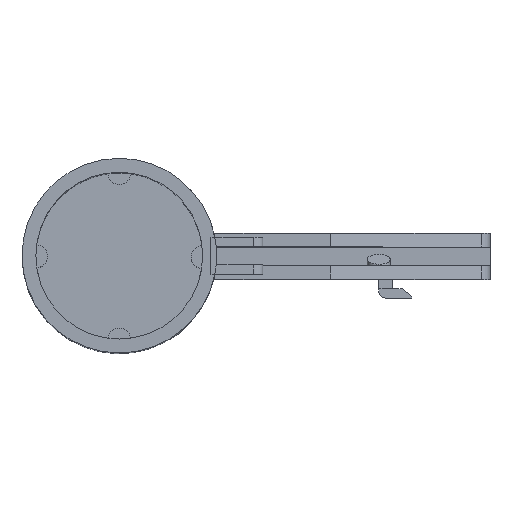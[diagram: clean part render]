
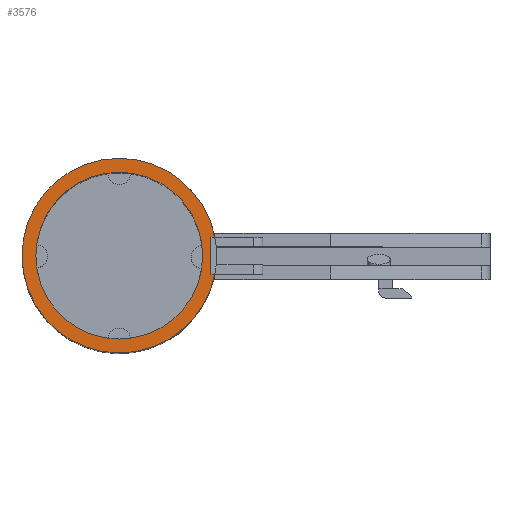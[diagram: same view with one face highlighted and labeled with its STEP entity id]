
A CAD part, top view. The second image highlights one B-rep face of the part: STEP entity #3576.
In plain terms, the highlighted planar face has unit normal (0, 0, 1).
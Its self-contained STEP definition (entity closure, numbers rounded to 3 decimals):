
#984 = CYLINDRICAL_SURFACE('',#985,21.);
#985 = AXIS2_PLACEMENT_3D('',#986,#987,#988);
#986 = CARTESIAN_POINT('',(0.,0.,0.));
#987 = DIRECTION('',(0.,0.,-1.));
#988 = DIRECTION('',(1.,0.,0.));
#2162 = VERTEX_POINT('',#2163);
#2163 = CARTESIAN_POINT('',(20.616,4.,100.));
#2187 = EDGE_CURVE('',#2162,#2188,#2190,.T.);
#2188 = VERTEX_POINT('',#2189);
#2189 = CARTESIAN_POINT('',(20.616,-4.,100.));
#2190 = SURFACE_CURVE('',#2191,(#2196,#2203),.PCURVE_S1.);
#2191 = CIRCLE('',#2192,21.);
#2192 = AXIS2_PLACEMENT_3D('',#2193,#2194,#2195);
#2193 = CARTESIAN_POINT('',(0.,0.,100.));
#2194 = DIRECTION('',(0.,0.,1.));
#2195 = DIRECTION('',(1.,0.,0.));
#2196 = PCURVE('',#984,#2197);
#2197 = DEFINITIONAL_REPRESENTATION('',(#2198),#2202);
#2198 = LINE('',#2199,#2200);
#2199 = CARTESIAN_POINT('',(0.,-100.));
#2200 = VECTOR('',#2201,1.);
#2201 = DIRECTION('',(-1.,0.));
#2202 = ( GEOMETRIC_REPRESENTATION_CONTEXT(2) 
PARAMETRIC_REPRESENTATION_CONTEXT() REPRESENTATION_CONTEXT('2D SPACE',''
  ) );
#2203 = PCURVE('',#2204,#2209);
#2204 = PLANE('',#2205);
#2205 = AXIS2_PLACEMENT_3D('',#2206,#2207,#2208);
#2206 = CARTESIAN_POINT('',(21.,0.,100.));
#2207 = DIRECTION('',(0.,0.,-1.));
#2208 = DIRECTION('',(-1.,0.,0.));
#2209 = DEFINITIONAL_REPRESENTATION('',(#2210),#2218);
#2210 = ( BOUNDED_CURVE() B_SPLINE_CURVE(2,(#2211,#2212,#2213,#2214,
#2215,#2216,#2217),.UNSPECIFIED.,.F.,.F.) B_SPLINE_CURVE_WITH_KNOTS((1,2
    ,2,2,2,1),(-2.094,0.,2.094,4.189,
6.283,8.378),.UNSPECIFIED.) CURVE() 
GEOMETRIC_REPRESENTATION_ITEM() RATIONAL_B_SPLINE_CURVE((1.,0.5,1.,0.5,
1.,0.5,1.)) REPRESENTATION_ITEM('') );
#2211 = CARTESIAN_POINT('',(0.,0.));
#2212 = CARTESIAN_POINT('',(0.,36.373));
#2213 = CARTESIAN_POINT('',(31.5,18.187));
#2214 = CARTESIAN_POINT('',(63.,0.));
#2215 = CARTESIAN_POINT('',(31.5,-18.187));
#2216 = CARTESIAN_POINT('',(0.,-36.373));
#2217 = CARTESIAN_POINT('',(0.,0.));
#2218 = ( GEOMETRIC_REPRESENTATION_CONTEXT(2) 
PARAMETRIC_REPRESENTATION_CONTEXT() REPRESENTATION_CONTEXT('2D SPACE',''
  ) );
#3576 = ADVANCED_FACE('',(#3577,#3652),#2204,.F.);
#3577 = FACE_BOUND('',#3578,.F.);
#3578 = EDGE_LOOP('',(#3579,#3580,#3608,#3631));
#3579 = ORIENTED_EDGE('',*,*,#2187,.F.);
#3580 = ORIENTED_EDGE('',*,*,#3581,.F.);
#3581 = EDGE_CURVE('',#3582,#2162,#3584,.T.);
#3582 = VERTEX_POINT('',#3583);
#3583 = CARTESIAN_POINT('',(19.777,4.,100.));
#3584 = SURFACE_CURVE('',#3585,(#3589,#3596),.PCURVE_S1.);
#3585 = LINE('',#3586,#3587);
#3586 = CARTESIAN_POINT('',(19.777,4.,100.));
#3587 = VECTOR('',#3588,1.);
#3588 = DIRECTION('',(1.,0.,0.));
#3589 = PCURVE('',#2204,#3590);
#3590 = DEFINITIONAL_REPRESENTATION('',(#3591),#3595);
#3591 = LINE('',#3592,#3593);
#3592 = CARTESIAN_POINT('',(1.223,4.));
#3593 = VECTOR('',#3594,1.);
#3594 = DIRECTION('',(-1.,0.));
#3595 = ( GEOMETRIC_REPRESENTATION_CONTEXT(2) 
PARAMETRIC_REPRESENTATION_CONTEXT() REPRESENTATION_CONTEXT('2D SPACE',''
  ) );
#3596 = PCURVE('',#3597,#3602);
#3597 = PLANE('',#3598);
#3598 = AXIS2_PLACEMENT_3D('',#3599,#3600,#3601);
#3599 = CARTESIAN_POINT('',(19.777,4.,100.));
#3600 = DIRECTION('',(0.,0.,1.));
#3601 = DIRECTION('',(1.,0.,0.));
#3602 = DEFINITIONAL_REPRESENTATION('',(#3603),#3607);
#3603 = LINE('',#3604,#3605);
#3604 = CARTESIAN_POINT('',(0.,0.));
#3605 = VECTOR('',#3606,1.);
#3606 = DIRECTION('',(1.,0.));
#3607 = ( GEOMETRIC_REPRESENTATION_CONTEXT(2) 
PARAMETRIC_REPRESENTATION_CONTEXT() REPRESENTATION_CONTEXT('2D SPACE',''
  ) );
#3608 = ORIENTED_EDGE('',*,*,#3609,.F.);
#3609 = EDGE_CURVE('',#3610,#3582,#3612,.T.);
#3610 = VERTEX_POINT('',#3611);
#3611 = CARTESIAN_POINT('',(19.777,-4.,100.));
#3612 = SURFACE_CURVE('',#3613,(#3617,#3624),.PCURVE_S1.);
#3613 = LINE('',#3614,#3615);
#3614 = CARTESIAN_POINT('',(19.777,-4.,100.));
#3615 = VECTOR('',#3616,1.);
#3616 = DIRECTION('',(0.,1.,0.));
#3617 = PCURVE('',#2204,#3618);
#3618 = DEFINITIONAL_REPRESENTATION('',(#3619),#3623);
#3619 = LINE('',#3620,#3621);
#3620 = CARTESIAN_POINT('',(1.223,-4.));
#3621 = VECTOR('',#3622,1.);
#3622 = DIRECTION('',(0.,1.));
#3623 = ( GEOMETRIC_REPRESENTATION_CONTEXT(2) 
PARAMETRIC_REPRESENTATION_CONTEXT() REPRESENTATION_CONTEXT('2D SPACE',''
  ) );
#3624 = PCURVE('',#3597,#3625);
#3625 = DEFINITIONAL_REPRESENTATION('',(#3626),#3630);
#3626 = LINE('',#3627,#3628);
#3627 = CARTESIAN_POINT('',(0.,-8.));
#3628 = VECTOR('',#3629,1.);
#3629 = DIRECTION('',(0.,1.));
#3630 = ( GEOMETRIC_REPRESENTATION_CONTEXT(2) 
PARAMETRIC_REPRESENTATION_CONTEXT() REPRESENTATION_CONTEXT('2D SPACE',''
  ) );
#3631 = ORIENTED_EDGE('',*,*,#3632,.F.);
#3632 = EDGE_CURVE('',#2188,#3610,#3633,.T.);
#3633 = SURFACE_CURVE('',#3634,(#3638,#3645),.PCURVE_S1.);
#3634 = LINE('',#3635,#3636);
#3635 = CARTESIAN_POINT('',(31.,-4.,100.));
#3636 = VECTOR('',#3637,1.);
#3637 = DIRECTION('',(-1.,0.,0.));
#3638 = PCURVE('',#2204,#3639);
#3639 = DEFINITIONAL_REPRESENTATION('',(#3640),#3644);
#3640 = LINE('',#3641,#3642);
#3641 = CARTESIAN_POINT('',(-10.,-4.));
#3642 = VECTOR('',#3643,1.);
#3643 = DIRECTION('',(1.,0.));
#3644 = ( GEOMETRIC_REPRESENTATION_CONTEXT(2) 
PARAMETRIC_REPRESENTATION_CONTEXT() REPRESENTATION_CONTEXT('2D SPACE',''
  ) );
#3645 = PCURVE('',#3597,#3646);
#3646 = DEFINITIONAL_REPRESENTATION('',(#3647),#3651);
#3647 = LINE('',#3648,#3649);
#3648 = CARTESIAN_POINT('',(11.223,-8.));
#3649 = VECTOR('',#3650,1.);
#3650 = DIRECTION('',(-1.,0.));
#3651 = ( GEOMETRIC_REPRESENTATION_CONTEXT(2) 
PARAMETRIC_REPRESENTATION_CONTEXT() REPRESENTATION_CONTEXT('2D SPACE',''
  ) );
#3652 = FACE_BOUND('',#3653,.F.);
#3653 = EDGE_LOOP('',(#3654));
#3654 = ORIENTED_EDGE('',*,*,#3655,.T.);
#3655 = EDGE_CURVE('',#3656,#3656,#3658,.T.);
#3656 = VERTEX_POINT('',#3657);
#3657 = CARTESIAN_POINT('',(18.,0.,100.));
#3658 = SURFACE_CURVE('',#3659,(#3664,#3675),.PCURVE_S1.);
#3659 = CIRCLE('',#3660,18.);
#3660 = AXIS2_PLACEMENT_3D('',#3661,#3662,#3663);
#3661 = CARTESIAN_POINT('',(0.,0.,100.));
#3662 = DIRECTION('',(0.,0.,1.));
#3663 = DIRECTION('',(1.,0.,0.));
#3664 = PCURVE('',#2204,#3665);
#3665 = DEFINITIONAL_REPRESENTATION('',(#3666),#3674);
#3666 = ( BOUNDED_CURVE() B_SPLINE_CURVE(2,(#3667,#3668,#3669,#3670,
#3671,#3672,#3673),.UNSPECIFIED.,.F.,.F.) B_SPLINE_CURVE_WITH_KNOTS((1,2
    ,2,2,2,1),(-2.094,0.,2.094,4.189,
6.283,8.378),.UNSPECIFIED.) CURVE() 
GEOMETRIC_REPRESENTATION_ITEM() RATIONAL_B_SPLINE_CURVE((1.,0.5,1.,0.5,
1.,0.5,1.)) REPRESENTATION_ITEM('') );
#3667 = CARTESIAN_POINT('',(3.,0.));
#3668 = CARTESIAN_POINT('',(3.,31.177));
#3669 = CARTESIAN_POINT('',(30.,15.588));
#3670 = CARTESIAN_POINT('',(57.,0.));
#3671 = CARTESIAN_POINT('',(30.,-15.588));
#3672 = CARTESIAN_POINT('',(3.,-31.177));
#3673 = CARTESIAN_POINT('',(3.,0.));
#3674 = ( GEOMETRIC_REPRESENTATION_CONTEXT(2) 
PARAMETRIC_REPRESENTATION_CONTEXT() REPRESENTATION_CONTEXT('2D SPACE',''
  ) );
#3675 = PCURVE('',#3676,#3681);
#3676 = CYLINDRICAL_SURFACE('',#3677,18.);
#3677 = AXIS2_PLACEMENT_3D('',#3678,#3679,#3680);
#3678 = CARTESIAN_POINT('',(0.,0.,100.));
#3679 = DIRECTION('',(0.,0.,1.));
#3680 = DIRECTION('',(1.,0.,0.));
#3681 = DEFINITIONAL_REPRESENTATION('',(#3682),#3686);
#3682 = LINE('',#3683,#3684);
#3683 = CARTESIAN_POINT('',(0.,0.));
#3684 = VECTOR('',#3685,1.);
#3685 = DIRECTION('',(1.,0.));
#3686 = ( GEOMETRIC_REPRESENTATION_CONTEXT(2) 
PARAMETRIC_REPRESENTATION_CONTEXT() REPRESENTATION_CONTEXT('2D SPACE',''
  ) );
